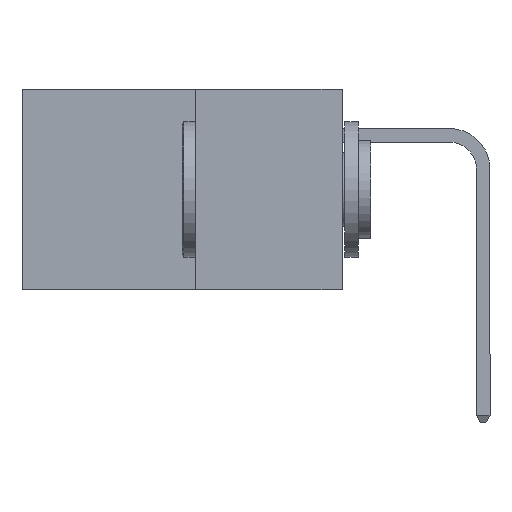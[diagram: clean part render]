
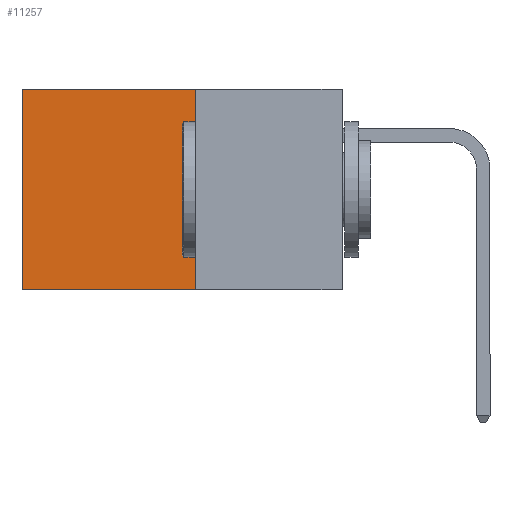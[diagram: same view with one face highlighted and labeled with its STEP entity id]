
A CAD part, left-side view. The second image highlights one B-rep face of the part: STEP entity #11257.
In plain terms, the highlighted planar face has unit normal (-1, 0, 0).
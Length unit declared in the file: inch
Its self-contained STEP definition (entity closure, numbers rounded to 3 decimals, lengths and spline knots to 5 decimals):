
#11 = VECTOR ( 'NONE', #5897, 39.37008 ) ;
#360 = VERTEX_POINT ( 'NONE', #3182 ) ;
#394 = FACE_OUTER_BOUND ( 'NONE', #5996, .T. ) ;
#792 = ORIENTED_EDGE ( 'NONE', *, *, #6961, .F. ) ;
#1196 = EDGE_CURVE ( 'NONE', #6069, #1251, #9069, .T. ) ;
#1244 = ORIENTED_EDGE ( 'NONE', *, *, #1196, .T. ) ;
#1251 = VERTEX_POINT ( 'NONE', #2687 ) ;
#1362 = VECTOR ( 'NONE', #9448, 39.37008 ) ;
#1801 = VECTOR ( 'NONE', #4502, 39.37008 ) ;
#2163 = ORIENTED_EDGE ( 'NONE', *, *, #7218, .F. ) ;
#2624 = CARTESIAN_POINT ( 'NONE',  ( 0.277, 0.27, -0.37 ) ) ;
#2687 = CARTESIAN_POINT ( 'NONE',  ( 0.277, 0.59, -0.37 ) ) ;
#3182 = CARTESIAN_POINT ( 'NONE',  ( 0.277, 0.27, 0. ) ) ;
#3650 = EDGE_CURVE ( 'NONE', #360, #6069, #8902, .T. ) ;
#3661 = CARTESIAN_POINT ( 'NONE',  ( 0.277, 0.59, 0. ) ) ;
#3676 = DIRECTION ( 'NONE',  ( 1., 0., 0. ) ) ;
#3913 = ORIENTED_EDGE ( 'NONE', *, *, #3650, .T. ) ;
#4502 = DIRECTION ( 'NONE',  ( 0., 0., -1. ) ) ;
#5019 = VERTEX_POINT ( 'NONE', #9039 ) ;
#5074 = LINE ( 'NONE', #5940, #11 ) ;
#5897 = DIRECTION ( 'NONE',  ( 0., 0., -1. ) ) ;
#5940 = CARTESIAN_POINT ( 'NONE',  ( 0.277, 0.27, -0.37 ) ) ;
#5996 = EDGE_LOOP ( 'NONE', ( #1244, #792, #2163, #3913 ) ) ;
#6069 = VERTEX_POINT ( 'NONE', #3661 ) ;
#6446 = CARTESIAN_POINT ( 'NONE',  ( 0.277, 0.59, -0.37 ) ) ;
#6548 = LINE ( 'NONE', #9501, #1362 ) ;
#6961 = EDGE_CURVE ( 'NONE', #5019, #1251, #6548, .T. ) ;
#7218 = EDGE_CURVE ( 'NONE', #360, #5019, #5074, .T. ) ;
#7964 = AXIS2_PLACEMENT_3D ( 'NONE', #2624, #3676, #10088 ) ;
#8297 = PLANE ( 'NONE',  #7964 ) ;
#8902 = LINE ( 'NONE', #11729, #10993 ) ;
#9039 = CARTESIAN_POINT ( 'NONE',  ( 0.277, 0.27, -0.37 ) ) ;
#9069 = LINE ( 'NONE', #6446, #1801 ) ;
#9448 = DIRECTION ( 'NONE',  ( 0., 1., 0. ) ) ;
#9501 = CARTESIAN_POINT ( 'NONE',  ( 0.277, 0.27, -0.37 ) ) ;
#10088 = DIRECTION ( 'NONE',  ( 0., 0., -1. ) ) ;
#10993 = VECTOR ( 'NONE', #11009, 39.37008 ) ;
#11009 = DIRECTION ( 'NONE',  ( 0., 1., 0. ) ) ;
#11257 = ADVANCED_FACE ( 'NONE', ( #394 ), #8297, .F. ) ;
#11729 = CARTESIAN_POINT ( 'NONE',  ( 0.277, 0.27, 0. ) ) ;
